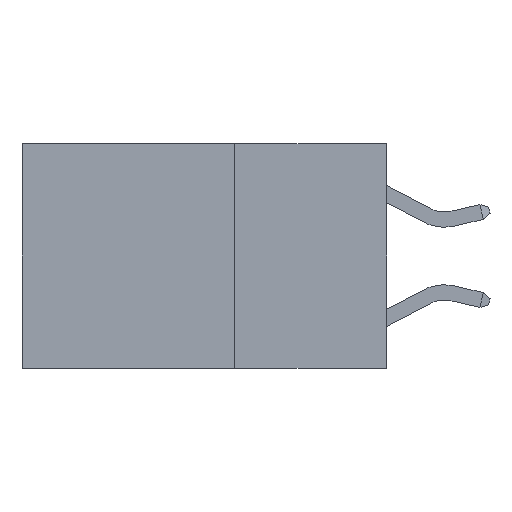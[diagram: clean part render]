
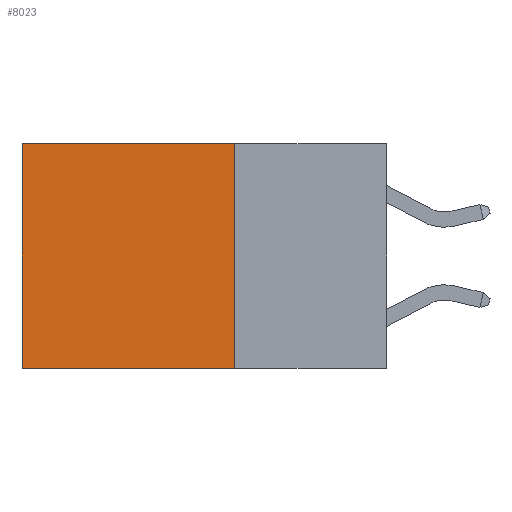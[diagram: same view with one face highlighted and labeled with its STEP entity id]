
A CAD part, left-side view. The second image highlights one B-rep face of the part: STEP entity #8023.
In plain terms, the highlighted planar face has unit normal (-1, 0, 0).
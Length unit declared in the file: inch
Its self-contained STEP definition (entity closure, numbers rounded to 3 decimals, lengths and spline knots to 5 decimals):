
#58 = EDGE_CURVE ( 'NONE', #14098, #11911, #10118, .T. ) ;
#215 = EDGE_CURVE ( 'NONE', #20583, #26479, #2555, .T. ) ;
#1038 = ORIENTED_EDGE ( 'NONE', *, *, #215, .T. ) ;
#1199 = VECTOR ( 'NONE', #27788, 39.37008 ) ;
#2263 = LINE ( 'NONE', #11080, #25052 ) ;
#2555 = LINE ( 'NONE', #7358, #7174 ) ;
#3394 = EDGE_CURVE ( 'NONE', #14098, #20583, #2263, .T. ) ;
#4173 = EDGE_CURVE ( 'NONE', #11911, #26479, #10727, .T. ) ;
#4740 = DIRECTION ( 'NONE',  ( 0., 0., -1. ) ) ;
#6255 = CARTESIAN_POINT ( 'NONE',  ( 0.2625, 0.25, -0.37 ) ) ;
#6328 = DIRECTION ( 'NONE',  ( 0., 1., 0. ) ) ;
#7174 = VECTOR ( 'NONE', #4740, 39.37008 ) ;
#7358 = CARTESIAN_POINT ( 'NONE',  ( 0.2625, 0.6, 0. ) ) ;
#8023 = ADVANCED_FACE ( 'NONE', ( #27072 ), #15902, .F. ) ;
#9080 = CARTESIAN_POINT ( 'NONE',  ( 0.2625, 0.6, 0. ) ) ;
#10078 = EDGE_LOOP ( 'NONE', ( #1038, #15716, #28447, #18188 ) ) ;
#10118 = LINE ( 'NONE', #14853, #1199 ) ;
#10727 = LINE ( 'NONE', #6255, #28320 ) ;
#11080 = CARTESIAN_POINT ( 'NONE',  ( 0.2625, 0.25, 0. ) ) ;
#11911 = VERTEX_POINT ( 'NONE', #20722 ) ;
#13466 = DIRECTION ( 'NONE',  ( 1., 0., 0. ) ) ;
#14098 = VERTEX_POINT ( 'NONE', #24196 ) ;
#14853 = CARTESIAN_POINT ( 'NONE',  ( 0.2625, 0.25, 0. ) ) ;
#15716 = ORIENTED_EDGE ( 'NONE', *, *, #4173, .F. ) ;
#15902 = PLANE ( 'NONE',  #26336 ) ;
#18188 = ORIENTED_EDGE ( 'NONE', *, *, #3394, .T. ) ;
#20583 = VERTEX_POINT ( 'NONE', #9080 ) ;
#20722 = CARTESIAN_POINT ( 'NONE',  ( 0.2625, 0.25, -0.37 ) ) ;
#21785 = CARTESIAN_POINT ( 'NONE',  ( 0.2625, 0.6, -0.37 ) ) ;
#24196 = CARTESIAN_POINT ( 'NONE',  ( 0.2625, 0.25, 0. ) ) ;
#24755 = CARTESIAN_POINT ( 'NONE',  ( 0.2625, 0.25, 0. ) ) ;
#25050 = DIRECTION ( 'NONE',  ( 0., 0., -1. ) ) ;
#25052 = VECTOR ( 'NONE', #6328, 39.37008 ) ;
#26253 = DIRECTION ( 'NONE',  ( 0., 1., 0. ) ) ;
#26336 = AXIS2_PLACEMENT_3D ( 'NONE', #24755, #13466, #25050 ) ;
#26479 = VERTEX_POINT ( 'NONE', #21785 ) ;
#27072 = FACE_OUTER_BOUND ( 'NONE', #10078, .T. ) ;
#27788 = DIRECTION ( 'NONE',  ( 0., 0., -1. ) ) ;
#28320 = VECTOR ( 'NONE', #26253, 39.37008 ) ;
#28447 = ORIENTED_EDGE ( 'NONE', *, *, #58, .F. ) ;
